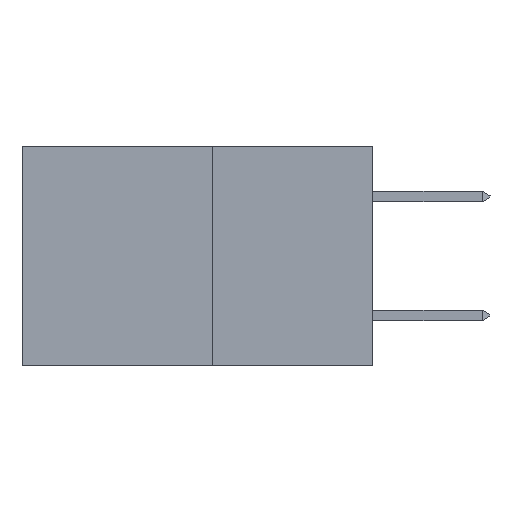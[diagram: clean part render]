
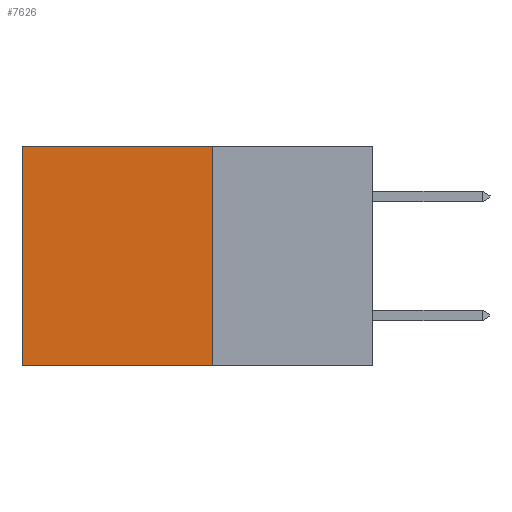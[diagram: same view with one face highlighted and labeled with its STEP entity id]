
A CAD part, left-side view. The second image highlights one B-rep face of the part: STEP entity #7626.
In plain terms, the highlighted planar face has unit normal (-1, 0, 0).
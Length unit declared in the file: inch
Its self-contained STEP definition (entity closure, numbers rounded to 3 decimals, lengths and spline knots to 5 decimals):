
#41 = DIRECTION ( 'NONE',  ( 0., 1., 0. ) ) ;
#198 = CARTESIAN_POINT ( 'NONE',  ( 0.277, 0.27, -0.37 ) ) ;
#497 = VERTEX_POINT ( 'NONE', #4041 ) ;
#1242 = EDGE_CURVE ( 'NONE', #5907, #497, #4152, .T. ) ;
#1526 = CARTESIAN_POINT ( 'NONE',  ( 0.277, 0.59, -0.37 ) ) ;
#1535 = CARTESIAN_POINT ( 'NONE',  ( 0.277, 0.27, 0. ) ) ;
#1616 = AXIS2_PLACEMENT_3D ( 'NONE', #5532, #2962, #7393 ) ;
#1827 = LINE ( 'NONE', #198, #5016 ) ;
#2027 = EDGE_CURVE ( 'NONE', #3548, #5083, #6112, .T. ) ;
#2847 = CARTESIAN_POINT ( 'NONE',  ( 0.277, 0.27, -0.37 ) ) ;
#2962 = DIRECTION ( 'NONE',  ( 1., 0., 0. ) ) ;
#3321 = EDGE_LOOP ( 'NONE', ( #3425, #3968, #4547, #7934 ) ) ;
#3364 = VECTOR ( 'NONE', #6787, 39.37008 ) ;
#3425 = ORIENTED_EDGE ( 'NONE', *, *, #3977, .T. ) ;
#3548 = VERTEX_POINT ( 'NONE', #2847 ) ;
#3820 = CARTESIAN_POINT ( 'NONE',  ( 0.277, 0.27, 0. ) ) ;
#3968 = ORIENTED_EDGE ( 'NONE', *, *, #2027, .F. ) ;
#3977 = EDGE_CURVE ( 'NONE', #497, #5083, #6711, .T. ) ;
#4041 = CARTESIAN_POINT ( 'NONE',  ( 0.277, 0.59, 0. ) ) ;
#4152 = LINE ( 'NONE', #1535, #5826 ) ;
#4547 = ORIENTED_EDGE ( 'NONE', *, *, #5956, .F. ) ;
#4896 = FACE_OUTER_BOUND ( 'NONE', #3321, .T. ) ;
#5016 = VECTOR ( 'NONE', #7700, 39.37008 ) ;
#5083 = VERTEX_POINT ( 'NONE', #6435 ) ;
#5532 = CARTESIAN_POINT ( 'NONE',  ( 0.277, 0.27, -0.37 ) ) ;
#5826 = VECTOR ( 'NONE', #6001, 39.37008 ) ;
#5907 = VERTEX_POINT ( 'NONE', #3820 ) ;
#5956 = EDGE_CURVE ( 'NONE', #5907, #3548, #1827, .T. ) ;
#6001 = DIRECTION ( 'NONE',  ( 0., 1., 0. ) ) ;
#6112 = LINE ( 'NONE', #7575, #8255 ) ;
#6435 = CARTESIAN_POINT ( 'NONE',  ( 0.277, 0.59, -0.37 ) ) ;
#6711 = LINE ( 'NONE', #1526, #3364 ) ;
#6753 = PLANE ( 'NONE',  #1616 ) ;
#6787 = DIRECTION ( 'NONE',  ( 0., 0., -1. ) ) ;
#7393 = DIRECTION ( 'NONE',  ( 0., 0., -1. ) ) ;
#7575 = CARTESIAN_POINT ( 'NONE',  ( 0.277, 0.27, -0.37 ) ) ;
#7626 = ADVANCED_FACE ( 'NONE', ( #4896 ), #6753, .F. ) ;
#7700 = DIRECTION ( 'NONE',  ( 0., 0., -1. ) ) ;
#7934 = ORIENTED_EDGE ( 'NONE', *, *, #1242, .T. ) ;
#8255 = VECTOR ( 'NONE', #41, 39.37008 ) ;
